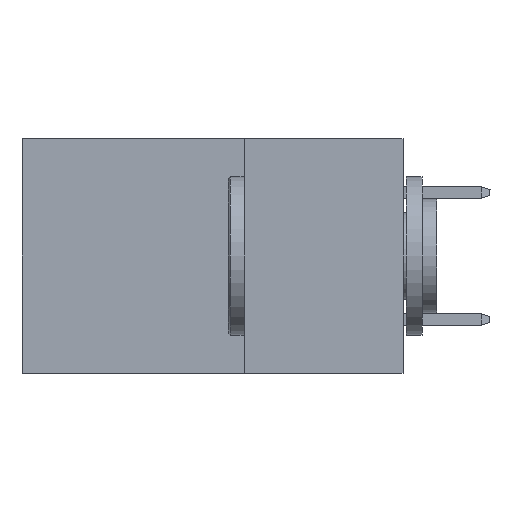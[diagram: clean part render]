
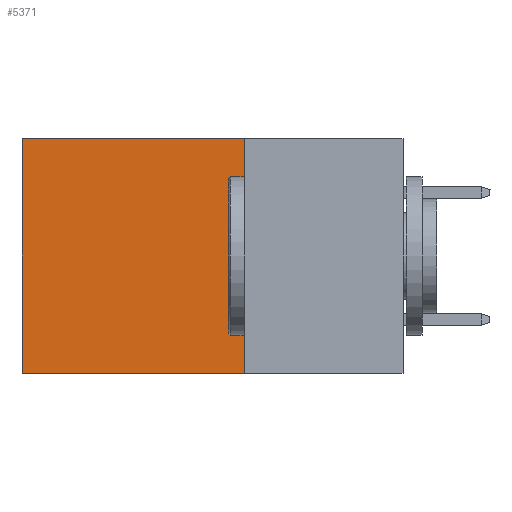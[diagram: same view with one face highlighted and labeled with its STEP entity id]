
A CAD part, left-side view. The second image highlights one B-rep face of the part: STEP entity #5371.
In plain terms, the highlighted planar face has unit normal (-1, 0, 0).
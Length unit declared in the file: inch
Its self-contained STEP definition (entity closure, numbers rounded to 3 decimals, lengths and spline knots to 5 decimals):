
#178 = PLANE ( 'NONE',  #10603 ) ;
#1814 = ORIENTED_EDGE ( 'NONE', *, *, #5686, .T. ) ;
#1921 = DIRECTION ( 'NONE',  ( 0., 0., -1. ) ) ;
#2456 = CARTESIAN_POINT ( 'NONE',  ( 0.2875, 0.25, -0.37 ) ) ;
#2854 = EDGE_CURVE ( 'NONE', #10963, #4265, #8786, .T. ) ;
#3559 = DIRECTION ( 'NONE',  ( 0., 1., 0. ) ) ;
#3848 = VERTEX_POINT ( 'NONE', #11459 ) ;
#4024 = DIRECTION ( 'NONE',  ( 0., 0., -1. ) ) ;
#4263 = VECTOR ( 'NONE', #4390, 39.37008 ) ;
#4265 = VERTEX_POINT ( 'NONE', #5841 ) ;
#4302 = ORIENTED_EDGE ( 'NONE', *, *, #2854, .F. ) ;
#4390 = DIRECTION ( 'NONE',  ( 0., 1., 0. ) ) ;
#4413 = EDGE_CURVE ( 'NONE', #10963, #3848, #9144, .T. ) ;
#4767 = CARTESIAN_POINT ( 'NONE',  ( 0.2875, 0.25, 0. ) ) ;
#4946 = ORIENTED_EDGE ( 'NONE', *, *, #6558, .F. ) ;
#5371 = ADVANCED_FACE ( 'NONE', ( #8689 ), #178, .F. ) ;
#5686 = EDGE_CURVE ( 'NONE', #3848, #11664, #12248, .T. ) ;
#5841 = CARTESIAN_POINT ( 'NONE',  ( 0.2875, 0.25, -0.37 ) ) ;
#6071 = VECTOR ( 'NONE', #7166, 39.37008 ) ;
#6558 = EDGE_CURVE ( 'NONE', #4265, #11664, #12056, .T. ) ;
#6583 = CARTESIAN_POINT ( 'NONE',  ( 0.2875, 0.6, -0.37 ) ) ;
#6902 = CARTESIAN_POINT ( 'NONE',  ( 0.2875, 0.25, 0. ) ) ;
#7166 = DIRECTION ( 'NONE',  ( 0., 0., -1. ) ) ;
#7203 = VECTOR ( 'NONE', #4024, 39.37008 ) ;
#7301 = CARTESIAN_POINT ( 'NONE',  ( 0.2875, 0.25, 0. ) ) ;
#7586 = DIRECTION ( 'NONE',  ( 1., 0., 0. ) ) ;
#8430 = CARTESIAN_POINT ( 'NONE',  ( 0.2875, 0.6, 0. ) ) ;
#8689 = FACE_OUTER_BOUND ( 'NONE', #11794, .T. ) ;
#8786 = LINE ( 'NONE', #4767, #7203 ) ;
#9144 = LINE ( 'NONE', #7301, #11946 ) ;
#9598 = ORIENTED_EDGE ( 'NONE', *, *, #4413, .T. ) ;
#10603 = AXIS2_PLACEMENT_3D ( 'NONE', #6902, #7586, #1921 ) ;
#10963 = VERTEX_POINT ( 'NONE', #11804 ) ;
#11459 = CARTESIAN_POINT ( 'NONE',  ( 0.2875, 0.6, 0. ) ) ;
#11664 = VERTEX_POINT ( 'NONE', #6583 ) ;
#11794 = EDGE_LOOP ( 'NONE', ( #1814, #4946, #4302, #9598 ) ) ;
#11804 = CARTESIAN_POINT ( 'NONE',  ( 0.2875, 0.25, 0. ) ) ;
#11946 = VECTOR ( 'NONE', #3559, 39.37008 ) ;
#12056 = LINE ( 'NONE', #2456, #4263 ) ;
#12248 = LINE ( 'NONE', #8430, #6071 ) ;
